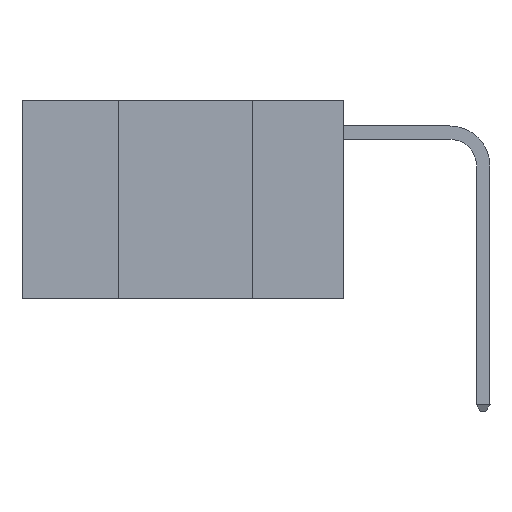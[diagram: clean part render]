
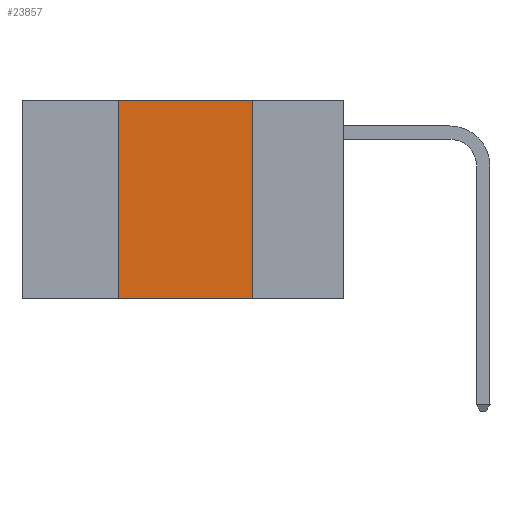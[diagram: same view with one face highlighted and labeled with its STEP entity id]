
A CAD part, left-side view. The second image highlights one B-rep face of the part: STEP entity #23857.
In plain terms, the highlighted planar face has unit normal (-1, 0, 0).
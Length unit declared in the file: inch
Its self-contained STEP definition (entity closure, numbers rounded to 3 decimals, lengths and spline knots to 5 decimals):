
#667 = VERTEX_POINT ( 'NONE', #7151 ) ;
#1050 = VERTEX_POINT ( 'NONE', #1513 ) ;
#1215 = VERTEX_POINT ( 'NONE', #25483 ) ;
#1513 = CARTESIAN_POINT ( 'NONE',  ( 0., 0.17, -0.37 ) ) ;
#1735 = DIRECTION ( 'NONE',  ( 0., -1., 0. ) ) ;
#4444 = EDGE_CURVE ( 'NONE', #22386, #1050, #19482, .T. ) ;
#4929 = FACE_OUTER_BOUND ( 'NONE', #10170, .T. ) ;
#5185 = CARTESIAN_POINT ( 'NONE',  ( 0., 0.6, 0. ) ) ;
#5379 = CARTESIAN_POINT ( 'NONE',  ( 0., 0.6, 0. ) ) ;
#5753 = LINE ( 'NONE', #13162, #11266 ) ;
#6937 = EDGE_CURVE ( 'NONE', #22386, #1215, #5753, .T. ) ;
#7151 = CARTESIAN_POINT ( 'NONE',  ( 0., 0.17, 0. ) ) ;
#8546 = DIRECTION ( 'NONE',  ( 0., 0., -1. ) ) ;
#8963 = CARTESIAN_POINT ( 'NONE',  ( 0., 0.42, -0.37 ) ) ;
#9051 = EDGE_CURVE ( 'NONE', #667, #1050, #25776, .T. ) ;
#9912 = PLANE ( 'NONE',  #12110 ) ;
#10170 = EDGE_LOOP ( 'NONE', ( #12857, #13618, #26798, #27881 ) ) ;
#11052 = CARTESIAN_POINT ( 'NONE',  ( 0., 0.6, -0.37 ) ) ;
#11266 = VECTOR ( 'NONE', #15503, 39.37008 ) ;
#12110 = AXIS2_PLACEMENT_3D ( 'NONE', #5185, #12254, #28663 ) ;
#12254 = DIRECTION ( 'NONE',  ( 1., 0., 0. ) ) ;
#12857 = ORIENTED_EDGE ( 'NONE', *, *, #9051, .F. ) ;
#13162 = CARTESIAN_POINT ( 'NONE',  ( 0., 0.42, 0. ) ) ;
#13256 = VECTOR ( 'NONE', #1735, 39.37008 ) ;
#13618 = ORIENTED_EDGE ( 'NONE', *, *, #26908, .F. ) ;
#15503 = DIRECTION ( 'NONE',  ( 0., 0., 1. ) ) ;
#19482 = LINE ( 'NONE', #11052, #13256 ) ;
#20230 = CARTESIAN_POINT ( 'NONE',  ( 0., 0.17, 0. ) ) ;
#21758 = DIRECTION ( 'NONE',  ( 0., -1., 0. ) ) ;
#22386 = VERTEX_POINT ( 'NONE', #8963 ) ;
#23091 = VECTOR ( 'NONE', #21758, 39.37008 ) ;
#23811 = LINE ( 'NONE', #5379, #23091 ) ;
#23857 = ADVANCED_FACE ( 'NONE', ( #4929 ), #9912, .F. ) ;
#25044 = VECTOR ( 'NONE', #8546, 39.37008 ) ;
#25483 = CARTESIAN_POINT ( 'NONE',  ( 0., 0.42, 0. ) ) ;
#25776 = LINE ( 'NONE', #20230, #25044 ) ;
#26798 = ORIENTED_EDGE ( 'NONE', *, *, #6937, .F. ) ;
#26908 = EDGE_CURVE ( 'NONE', #1215, #667, #23811, .T. ) ;
#27881 = ORIENTED_EDGE ( 'NONE', *, *, #4444, .T. ) ;
#28663 = DIRECTION ( 'NONE',  ( 0., 0., -1. ) ) ;
